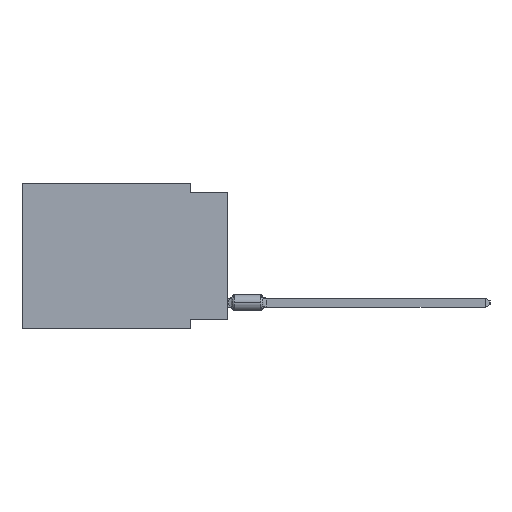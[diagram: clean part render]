
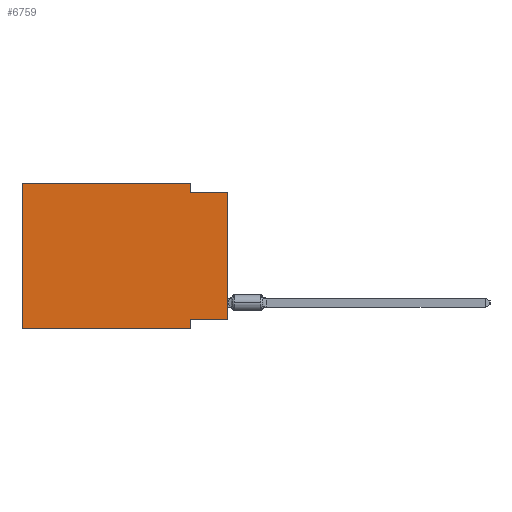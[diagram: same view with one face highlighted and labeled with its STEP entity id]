
A CAD part, left-side view. The second image highlights one B-rep face of the part: STEP entity #6759.
In plain terms, the highlighted planar face has unit normal (-1, 0, 0).
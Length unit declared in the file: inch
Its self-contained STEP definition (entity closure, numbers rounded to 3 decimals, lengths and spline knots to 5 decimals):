
#271 = LINE ( 'NONE', #43475, #46227 ) ;
#610 = DIRECTION ( 'NONE',  ( 0., 0., 1. ) ) ;
#1032 = LINE ( 'NONE', #6255, #54250 ) ;
#1067 = ORIENTED_EDGE ( 'NONE', *, *, #57936, .F. ) ;
#2405 = DIRECTION ( 'NONE',  ( 0., 1., 0. ) ) ;
#3064 = CARTESIAN_POINT ( 'NONE',  ( 0., 0.55, 0. ) ) ;
#3376 = EDGE_CURVE ( 'NONE', #67770, #64078, #50960, .T. ) ;
#3945 = DIRECTION ( 'NONE',  ( 0., -1., 0. ) ) ;
#4449 = ORIENTED_EDGE ( 'NONE', *, *, #3376, .F. ) ;
#6255 = CARTESIAN_POINT ( 'NONE',  ( 0., 0., -0.365 ) ) ;
#6480 = VECTOR ( 'NONE', #65914, 39.37008 ) ;
#6750 = CARTESIAN_POINT ( 'NONE',  ( 0., 0.1, -0.365 ) ) ;
#6759 = ADVANCED_FACE ( 'NONE', ( #24767 ), #14651, .F. ) ;
#12668 = DIRECTION ( 'NONE',  ( 0., -1., 0. ) ) ;
#13649 = DIRECTION ( 'NONE',  ( 0., 0., 1. ) ) ;
#14651 = PLANE ( 'NONE',  #36933 ) ;
#15342 = EDGE_CURVE ( 'NONE', #63179, #25840, #36262, .T. ) ;
#15733 = DIRECTION ( 'NONE',  ( 0., 0., -1. ) ) ;
#20016 = CARTESIAN_POINT ( 'NONE',  ( 0., 0.1, 0. ) ) ;
#23586 = ORIENTED_EDGE ( 'NONE', *, *, #15342, .F. ) ;
#24060 = CARTESIAN_POINT ( 'NONE',  ( 0., 0.1, 0. ) ) ;
#24447 = CARTESIAN_POINT ( 'NONE',  ( 0., 0., -0.025 ) ) ;
#24767 = FACE_OUTER_BOUND ( 'NONE', #52946, .T. ) ;
#25840 = VERTEX_POINT ( 'NONE', #3064 ) ;
#29503 = EDGE_CURVE ( 'NONE', #25840, #48057, #55896, .T. ) ;
#31913 = ORIENTED_EDGE ( 'NONE', *, *, #29503, .F. ) ;
#33148 = CARTESIAN_POINT ( 'NONE',  ( 0., 0.55, -0.39 ) ) ;
#34317 = ORIENTED_EDGE ( 'NONE', *, *, #65838, .F. ) ;
#34888 = ORIENTED_EDGE ( 'NONE', *, *, #42853, .F. ) ;
#35188 = CARTESIAN_POINT ( 'NONE',  ( 0., 0.1, -0.025 ) ) ;
#35902 = CARTESIAN_POINT ( 'NONE',  ( 0., 0.55, 0. ) ) ;
#36262 = LINE ( 'NONE', #41490, #62579 ) ;
#36933 = AXIS2_PLACEMENT_3D ( 'NONE', #35902, #57192, #46043 ) ;
#38439 = VECTOR ( 'NONE', #12668, 39.37008 ) ;
#39317 = VERTEX_POINT ( 'NONE', #6750 ) ;
#39813 = VECTOR ( 'NONE', #3945, 39.37008 ) ;
#40225 = VECTOR ( 'NONE', #15733, 39.37008 ) ;
#40567 = EDGE_CURVE ( 'NONE', #54916, #64078, #271, .T. ) ;
#40815 = DIRECTION ( 'NONE',  ( 0., -1., 0. ) ) ;
#41490 = CARTESIAN_POINT ( 'NONE',  ( 0., 0.55, 0. ) ) ;
#42632 = CARTESIAN_POINT ( 'NONE',  ( 0., 0., -0.365 ) ) ;
#42853 = EDGE_CURVE ( 'NONE', #54916, #39317, #1032, .T. ) ;
#43064 = ORIENTED_EDGE ( 'NONE', *, *, #45022, .T. ) ;
#43475 = CARTESIAN_POINT ( 'NONE',  ( 0., 0., 0. ) ) ;
#44996 = LINE ( 'NONE', #24060, #6480 ) ;
#45022 = EDGE_CURVE ( 'NONE', #63179, #57285, #56957, .T. ) ;
#46043 = DIRECTION ( 'NONE',  ( 0., 0., -1. ) ) ;
#46227 = VECTOR ( 'NONE', #610, 39.37008 ) ;
#48057 = VERTEX_POINT ( 'NONE', #20016 ) ;
#48840 = LINE ( 'NONE', #63493, #40225 ) ;
#50473 = CARTESIAN_POINT ( 'NONE',  ( 0., 0.1, -0.39 ) ) ;
#50960 = LINE ( 'NONE', #24447, #65073 ) ;
#52946 = EDGE_LOOP ( 'NONE', ( #58174, #4449, #1067, #31913, #23586, #43064, #34317, #34888 ) ) ;
#54250 = VECTOR ( 'NONE', #2405, 39.37008 ) ;
#54916 = VERTEX_POINT ( 'NONE', #42632 ) ;
#55896 = LINE ( 'NONE', #60453, #38439 ) ;
#56957 = LINE ( 'NONE', #66728, #39813 ) ;
#57192 = DIRECTION ( 'NONE',  ( 1., 0., 0. ) ) ;
#57285 = VERTEX_POINT ( 'NONE', #50473 ) ;
#57936 = EDGE_CURVE ( 'NONE', #48057, #67770, #44996, .T. ) ;
#58174 = ORIENTED_EDGE ( 'NONE', *, *, #40567, .T. ) ;
#60453 = CARTESIAN_POINT ( 'NONE',  ( 0., 0.55, 0. ) ) ;
#62579 = VECTOR ( 'NONE', #13649, 39.37008 ) ;
#63179 = VERTEX_POINT ( 'NONE', #33148 ) ;
#63493 = CARTESIAN_POINT ( 'NONE',  ( 0., 0.1, -0.39 ) ) ;
#64078 = VERTEX_POINT ( 'NONE', #66084 ) ;
#65073 = VECTOR ( 'NONE', #40815, 39.37008 ) ;
#65838 = EDGE_CURVE ( 'NONE', #39317, #57285, #48840, .T. ) ;
#65914 = DIRECTION ( 'NONE',  ( 0., 0., -1. ) ) ;
#66084 = CARTESIAN_POINT ( 'NONE',  ( 0., 0., -0.025 ) ) ;
#66728 = CARTESIAN_POINT ( 'NONE',  ( 0., 0.55, -0.39 ) ) ;
#67770 = VERTEX_POINT ( 'NONE', #35188 ) ;
